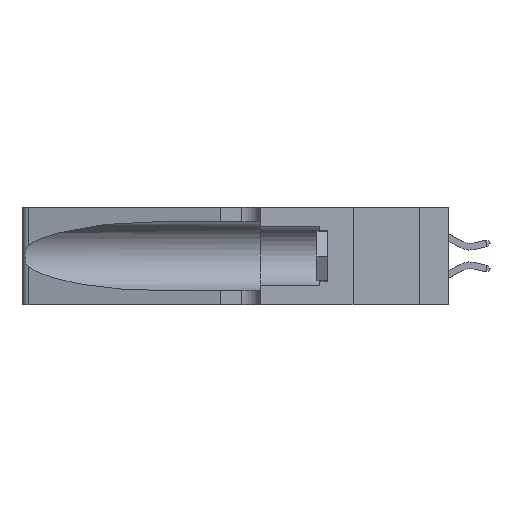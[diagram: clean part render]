
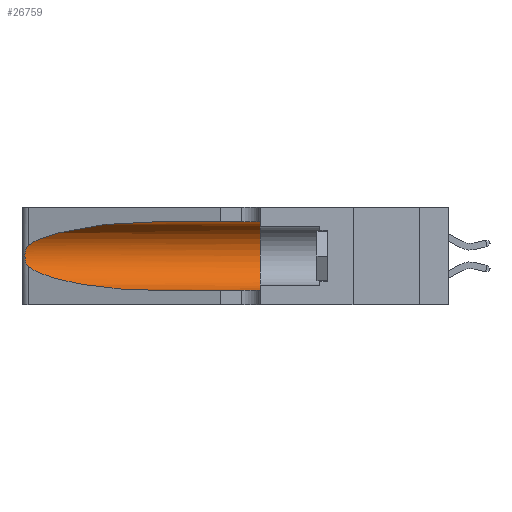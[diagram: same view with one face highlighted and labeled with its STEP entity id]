
A CAD part, left-side view. The second image highlights one B-rep face of the part: STEP entity #26759.
In plain terms, the highlighted cylindrical face has radius 3.308 mm (diameter 6.617 mm), a partial arc.
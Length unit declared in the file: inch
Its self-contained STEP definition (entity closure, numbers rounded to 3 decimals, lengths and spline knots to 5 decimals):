
#291 = CARTESIAN_POINT ( 'NONE',  ( 0.25555, 1.22994, 0.2215 ) ) ;
#520 = VERTEX_POINT ( 'NONE', #25201 ) ;
#598 = DIRECTION ( 'NONE',  ( 0., 1., 0. ) ) ;
#656 = CARTESIAN_POINT ( 'NONE',  ( 0.25787, 1.23484, 0.2124 ) ) ;
#764 = DIRECTION ( 'NONE',  ( 0., -1., 0. ) ) ;
#892 = CARTESIAN_POINT ( 'NONE',  ( 0.1305, 1.61858, 0.185 ) ) ;
#948 = CARTESIAN_POINT ( 'NONE',  ( 0.2373, 1.15595, 0.08982 ) ) ;
#1002 = CARTESIAN_POINT ( 'NONE',  ( 0.26075, 1.23896, 0.178 ) ) ;
#1168 = CARTESIAN_POINT ( 'NONE',  ( 0.25854, 1.2359, 0.20912 ) ) ;
#1321 = CARTESIAN_POINT ( 'NONE',  ( 0.1305, 1.61858, 0.05475 ) ) ;
#1633 = CARTESIAN_POINT ( 'NONE',  ( 0.25856, 1.23593, 0.16098 ) ) ;
#1937 = CARTESIAN_POINT ( 'NONE',  ( 0.25639, 1.23186, 0.15144 ) ) ;
#2537 = EDGE_CURVE ( 'NONE', #17190, #33062, #12833, .T. ) ;
#3267 = CARTESIAN_POINT ( 'NONE',  ( 0.25487, 1.22718, 0.22369 ) ) ;
#3511 = CARTESIAN_POINT ( 'NONE',  ( 0.2373, 1.15595, 0.28018 ) ) ;
#3712 = EDGE_CURVE ( 'NONE', #31800, #27631, #4871, .T. ) ;
#4871 =( BOUNDED_CURVE ( )  B_SPLINE_CURVE ( 3, ( #33993, #34225, #3511, #28501 ),
 .UNSPECIFIED., .F., .F. ) 
 B_SPLINE_CURVE_WITH_KNOTS ( ( 4, 4 ),
 ( 1.5708, 2.84003 ),
 .UNSPECIFIED. ) 
 CURVE ( )  GEOMETRIC_REPRESENTATION_ITEM ( )  RATIONAL_B_SPLINE_CURVE ( ( 1., 0.87, 0.87, 1. ) ) 
 REPRESENTATION_ITEM ( '' )  );
#5549 = CARTESIAN_POINT ( 'NONE',  ( 0.26075, 1.23896, 0.19203 ) ) ;
#6759 = EDGE_CURVE ( 'NONE', #520, #17190, #35051, .T. ) ;
#7017 = CARTESIAN_POINT ( 'NONE',  ( 0.26017, 1.23833, 0.17102 ) ) ;
#8685 = B_SPLINE_CURVE_WITH_KNOTS ( 'NONE', 3,
 ( #3267, #291, #30941, #656, #1168, #35783, #5549, #1002, #7017, #1633, #21885, #1937, #35466, #10575 ),
 .UNSPECIFIED., .F., .F.,
 ( 4, 2, 2, 2, 2, 2, 4 ),
 ( 0., 0.00027, 0.00053, 0.00107, 0.0016, 0.00187, 0.00214 ),
 .UNSPECIFIED. ) ;
#9347 = ORIENTED_EDGE ( 'NONE', *, *, #6759, .T. ) ;
#10575 = CARTESIAN_POINT ( 'NONE',  ( 0.25487, 1.22718, 0.14631 ) ) ;
#10870 = CARTESIAN_POINT ( 'NONE',  ( 0.1305, 0.72297, 0.05475 ) ) ;
#10960 = EDGE_CURVE ( 'NONE', #27631, #520, #8685, .T. ) ;
#11780 = EDGE_CURVE ( 'NONE', #34952, #33062, #13689, .T. ) ;
#11971 = DIRECTION ( 'NONE',  ( 0., 0., -1. ) ) ;
#12148 = CARTESIAN_POINT ( 'NONE',  ( 0.25487, 1.22718, 0.14631 ) ) ;
#12285 = FACE_OUTER_BOUND ( 'NONE', #16631, .T. ) ;
#12833 = LINE ( 'NONE', #1321, #23716 ) ;
#13689 = CIRCLE ( 'NONE', #32095, 0.13025 ) ;
#14290 = DIRECTION ( 'NONE',  ( 0., 0., 1. ) ) ;
#16631 = EDGE_LOOP ( 'NONE', ( #28385, #32752, #9347, #16828, #20238, #25671 ) ) ;
#16828 = ORIENTED_EDGE ( 'NONE', *, *, #2537, .T. ) ;
#17190 = VERTEX_POINT ( 'NONE', #10870 ) ;
#18313 = CARTESIAN_POINT ( 'NONE',  ( 0.1305, 0.35, 0.05475 ) ) ;
#19529 = VECTOR ( 'NONE', #21722, 39.37008 ) ;
#20238 = ORIENTED_EDGE ( 'NONE', *, *, #11780, .F. ) ;
#20411 = CARTESIAN_POINT ( 'NONE',  ( 0.18966, 0.96281, 0.05475 ) ) ;
#20815 = AXIS2_PLACEMENT_3D ( 'NONE', #892, #764, #11971 ) ;
#20919 = CARTESIAN_POINT ( 'NONE',  ( 0.25487, 1.22718, 0.22369 ) ) ;
#21722 = DIRECTION ( 'NONE',  ( 0., -1., 0. ) ) ;
#21885 = CARTESIAN_POINT ( 'NONE',  ( 0.25789, 1.23486, 0.15765 ) ) ;
#23197 = CARTESIAN_POINT ( 'NONE',  ( 0.1305, 0.72297, 0.05475 ) ) ;
#23716 = VECTOR ( 'NONE', #24424, 39.37008 ) ;
#24424 = DIRECTION ( 'NONE',  ( 0., -1., 0. ) ) ;
#25201 = CARTESIAN_POINT ( 'NONE',  ( 0.25487, 1.22718, 0.14631 ) ) ;
#25671 = ORIENTED_EDGE ( 'NONE', *, *, #30257, .F. ) ;
#26759 = ADVANCED_FACE ( 'NONE', ( #12285 ), #31073, .F. ) ;
#27631 = VERTEX_POINT ( 'NONE', #20919 ) ;
#28385 = ORIENTED_EDGE ( 'NONE', *, *, #3712, .T. ) ;
#28501 = CARTESIAN_POINT ( 'NONE',  ( 0.25487, 1.22718, 0.22369 ) ) ;
#29961 = CARTESIAN_POINT ( 'NONE',  ( 0.1305, 1.61858, 0.31525 ) ) ;
#30257 = EDGE_CURVE ( 'NONE', #31800, #34952, #31342, .T. ) ;
#30941 = CARTESIAN_POINT ( 'NONE',  ( 0.25639, 1.23184, 0.21858 ) ) ;
#31073 = CYLINDRICAL_SURFACE ( 'NONE', #20815, 0.13025 ) ;
#31247 = CARTESIAN_POINT ( 'NONE',  ( 0.1305, 0.35, 0.185 ) ) ;
#31342 = LINE ( 'NONE', #29961, #19529 ) ;
#31800 = VERTEX_POINT ( 'NONE', #35992 ) ;
#32095 = AXIS2_PLACEMENT_3D ( 'NONE', #31247, #598, #14290 ) ;
#32752 = ORIENTED_EDGE ( 'NONE', *, *, #10960, .T. ) ;
#33062 = VERTEX_POINT ( 'NONE', #18313 ) ;
#33536 = CARTESIAN_POINT ( 'NONE',  ( 0.1305, 0.35, 0.31525 ) ) ;
#33993 = CARTESIAN_POINT ( 'NONE',  ( 0.1305, 0.72297, 0.31525 ) ) ;
#34225 = CARTESIAN_POINT ( 'NONE',  ( 0.18966, 0.96281, 0.31525 ) ) ;
#34952 = VERTEX_POINT ( 'NONE', #33536 ) ;
#35051 =( BOUNDED_CURVE ( )  B_SPLINE_CURVE ( 3, ( #12148, #948, #20411, #23197 ),
 .UNSPECIFIED., .F., .F. ) 
 B_SPLINE_CURVE_WITH_KNOTS ( ( 4, 4 ),
 ( 3.44316, 4.71239 ),
 .UNSPECIFIED. ) 
 CURVE ( )  GEOMETRIC_REPRESENTATION_ITEM ( )  RATIONAL_B_SPLINE_CURVE ( ( 1., 0.87, 0.87, 1. ) ) 
 REPRESENTATION_ITEM ( '' )  );
#35466 = CARTESIAN_POINT ( 'NONE',  ( 0.25555, 1.22993, 0.14849 ) ) ;
#35783 = CARTESIAN_POINT ( 'NONE',  ( 0.26018, 1.23835, 0.19895 ) ) ;
#35992 = CARTESIAN_POINT ( 'NONE',  ( 0.1305, 0.72297, 0.31525 ) ) ;
